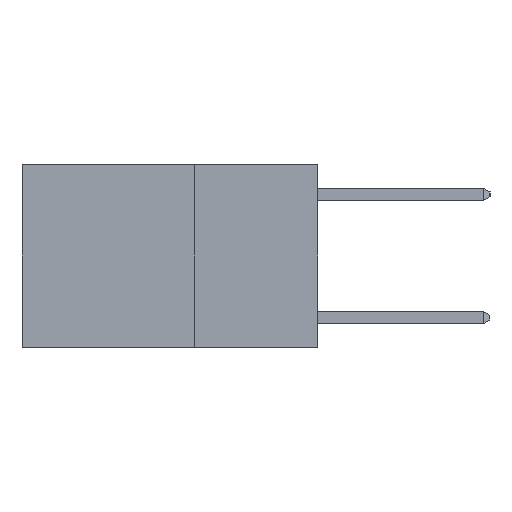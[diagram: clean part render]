
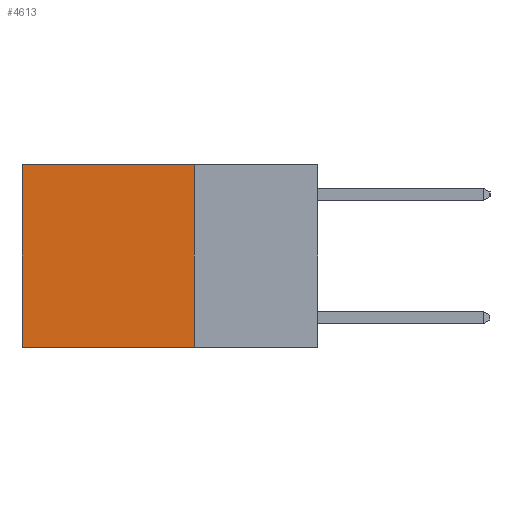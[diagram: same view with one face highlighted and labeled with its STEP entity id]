
A CAD part, left-side view. The second image highlights one B-rep face of the part: STEP entity #4613.
In plain terms, the highlighted planar face has unit normal (-1, 0, 0).
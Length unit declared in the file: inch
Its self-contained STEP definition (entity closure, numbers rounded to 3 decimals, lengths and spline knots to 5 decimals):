
#104 = CARTESIAN_POINT ( 'NONE',  ( 0.2625, 0.25, -0.37 ) ) ;
#603 = EDGE_CURVE ( 'NONE', #7602, #754, #852, .T. ) ;
#630 = EDGE_CURVE ( 'NONE', #7749, #754, #8450, .T. ) ;
#719 = VECTOR ( 'NONE', #9320, 39.37008 ) ;
#754 = VERTEX_POINT ( 'NONE', #8956 ) ;
#852 = LINE ( 'NONE', #10450, #4785 ) ;
#954 = CARTESIAN_POINT ( 'NONE',  ( 0.2625, 0.6, 0. ) ) ;
#1123 = VERTEX_POINT ( 'NONE', #8163 ) ;
#1867 = DIRECTION ( 'NONE',  ( 1., 0., 0. ) ) ;
#2290 = AXIS2_PLACEMENT_3D ( 'NONE', #7015, #1867, #7829 ) ;
#2891 = ORIENTED_EDGE ( 'NONE', *, *, #630, .T. ) ;
#3221 = DIRECTION ( 'NONE',  ( 0., 0., -1. ) ) ;
#4187 = EDGE_LOOP ( 'NONE', ( #2891, #4913, #4543, #6549 ) ) ;
#4543 = ORIENTED_EDGE ( 'NONE', *, *, #7984, .F. ) ;
#4613 = ADVANCED_FACE ( 'NONE', ( #6824 ), #9464, .F. ) ;
#4785 = VECTOR ( 'NONE', #10908, 39.37008 ) ;
#4913 = ORIENTED_EDGE ( 'NONE', *, *, #603, .F. ) ;
#6260 = VECTOR ( 'NONE', #3221, 39.37008 ) ;
#6549 = ORIENTED_EDGE ( 'NONE', *, *, #10397, .T. ) ;
#6654 = CARTESIAN_POINT ( 'NONE',  ( 0.2625, 0.25, 0. ) ) ;
#6824 = FACE_OUTER_BOUND ( 'NONE', #4187, .T. ) ;
#7015 = CARTESIAN_POINT ( 'NONE',  ( 0.2625, 0.25, 0. ) ) ;
#7602 = VERTEX_POINT ( 'NONE', #104 ) ;
#7610 = LINE ( 'NONE', #8463, #719 ) ;
#7749 = VERTEX_POINT ( 'NONE', #8904 ) ;
#7829 = DIRECTION ( 'NONE',  ( 0., 0., -1. ) ) ;
#7984 = EDGE_CURVE ( 'NONE', #1123, #7602, #7610, .T. ) ;
#8163 = CARTESIAN_POINT ( 'NONE',  ( 0.2625, 0.25, 0. ) ) ;
#8315 = DIRECTION ( 'NONE',  ( 0., 1., 0. ) ) ;
#8450 = LINE ( 'NONE', #954, #6260 ) ;
#8463 = CARTESIAN_POINT ( 'NONE',  ( 0.2625, 0.25, 0. ) ) ;
#8468 = VECTOR ( 'NONE', #8315, 39.37008 ) ;
#8904 = CARTESIAN_POINT ( 'NONE',  ( 0.2625, 0.6, 0. ) ) ;
#8956 = CARTESIAN_POINT ( 'NONE',  ( 0.2625, 0.6, -0.37 ) ) ;
#9320 = DIRECTION ( 'NONE',  ( 0., 0., -1. ) ) ;
#9464 = PLANE ( 'NONE',  #2290 ) ;
#10397 = EDGE_CURVE ( 'NONE', #1123, #7749, #10878, .T. ) ;
#10450 = CARTESIAN_POINT ( 'NONE',  ( 0.2625, 0.25, -0.37 ) ) ;
#10878 = LINE ( 'NONE', #6654, #8468 ) ;
#10908 = DIRECTION ( 'NONE',  ( 0., 1., 0. ) ) ;
